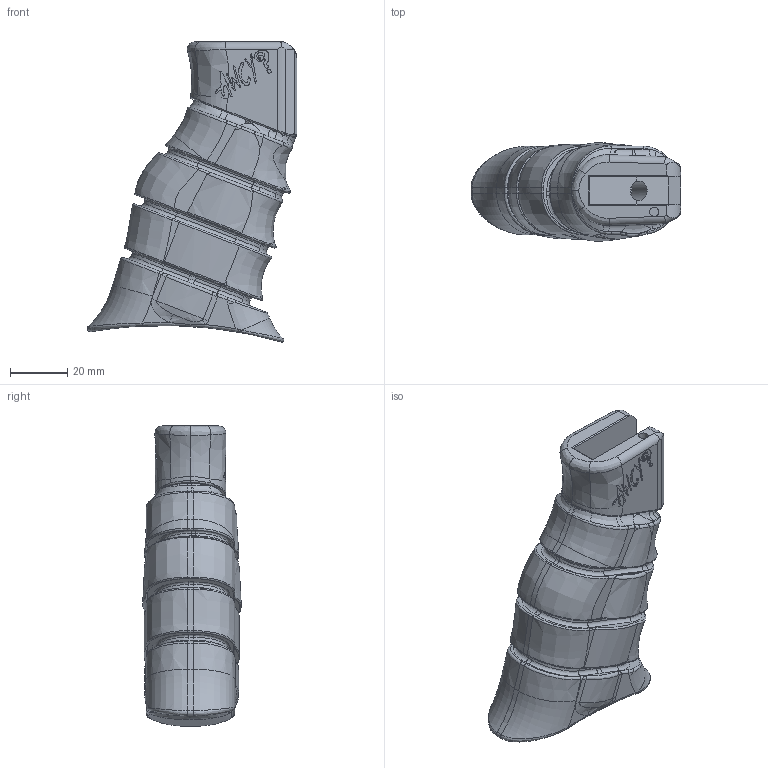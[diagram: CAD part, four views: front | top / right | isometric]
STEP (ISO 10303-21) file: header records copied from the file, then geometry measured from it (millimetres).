
FILE_DESCRIPTION(('STEP AP214'),'1');
FILE_NAME('AR15- AKaBar Grip.stp','2021-07-13T17:31:06',(' '),(' '),'Spatial InterOp 3D',' ',' ');
FILE_SCHEMA(('AUTOMOTIVE_DESIGN { 1 0 10303 214 1 1 1 1 }'));
Length unit declared in the file: metre
Products named in the file (1): revised kabar grip full assembly
Bounding box: 72.9 x 34.33 x 104.42 mm (x, y, z)
Volume: 79070.8 mm3; surface area: 27593.7 mm2
Topology: 1 solids, 1 shells, 878 faces, 2441 edges, 1565 vertices
Faces by surface type: plane 262, bspline 238, extrusion 223, cylinder 128, torus 23, cone 4
Full cylindrical faces by diameter (mm): 3.231 x1, 6.8 x1
Entity records: 104954 total; most frequent: CARTESIAN_POINT 84883, ORIENTED_EDGE 4842, DIRECTION 2944, EDGE_CURVE 2421, VERTEX_POINT 1565, VECTOR 1234, B_SPLINE_CURVE_WITH_KNOTS 1195, LINE 1011
